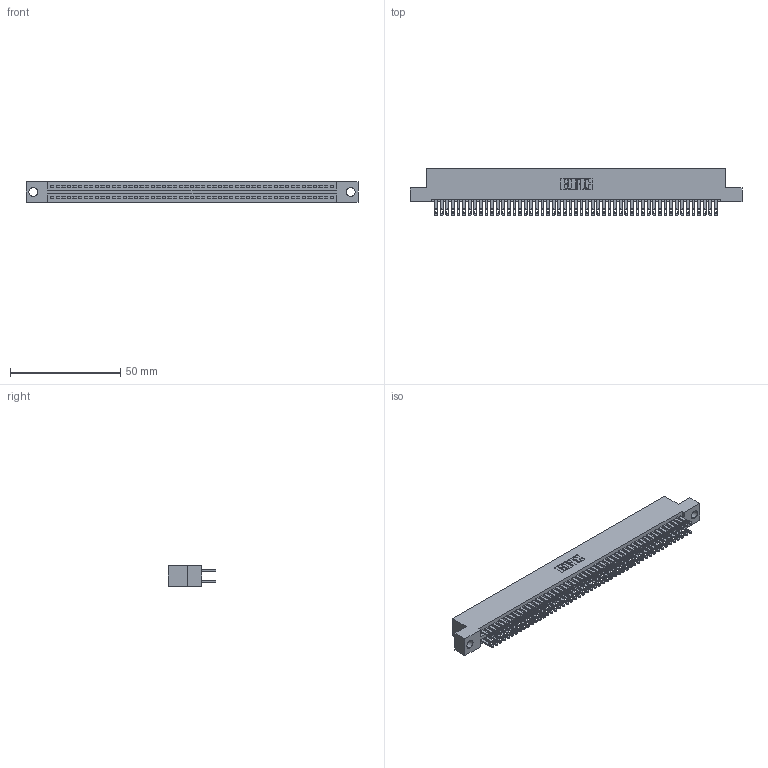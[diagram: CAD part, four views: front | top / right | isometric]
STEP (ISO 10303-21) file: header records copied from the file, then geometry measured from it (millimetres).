
FILE_DESCRIPTION (( 'STEP AP203' ), '1' );
FILE_NAME ('345-102-500-204.STEP', '2018-10-05T18:20:43', ( '' ), ( '' ), 'SwSTEP 2.0', 'SolidWorks 2016', '' );
FILE_SCHEMA (( 'CONFIG_CONTROL_DESIGN' ));
Length unit declared in the file: inch
Products named in the file (3): 345-292-001_345-293-100; 345 Part_Flush Mounting Lugs - 0.156 Dia-TH; 345-102-500-204
Assembly tree (103 placements, depth 2):
  345-102-500-204
    345 Part_Flush Mounting Lugs - 0.156 Dia-TH
    345-292-001_345-293-100  x102
Bounding box: 150.75 x 21.51 x 9.4 mm (x, y, z)
Volume: 14951.3 mm3; surface area: 23130.3 mm2
Topology: 103 solids, 103 shells, 4818 faces, 14723 edges, 9814 vertices
Faces by surface type: plane 2834, cylinder 1984
Entity records: 38737 total; most frequent: CARTESIAN_POINT 6484, ORIENTED_EDGE 6418, DIRECTION 5709, EDGE_CURVE 3209, LINE 2869, VECTOR 2869, VERTEX_POINT 2138, AXIS2_PLACEMENT_3D 1420
